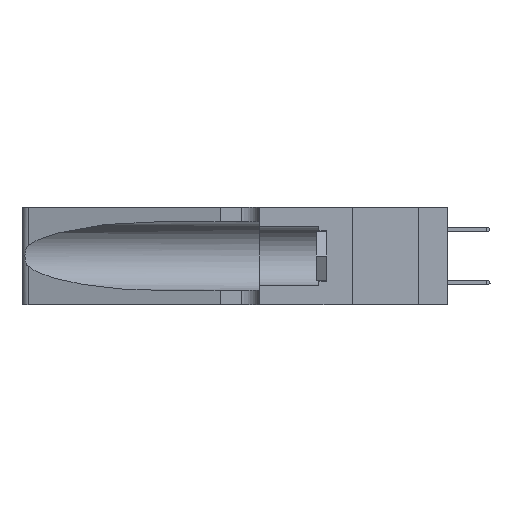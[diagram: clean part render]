
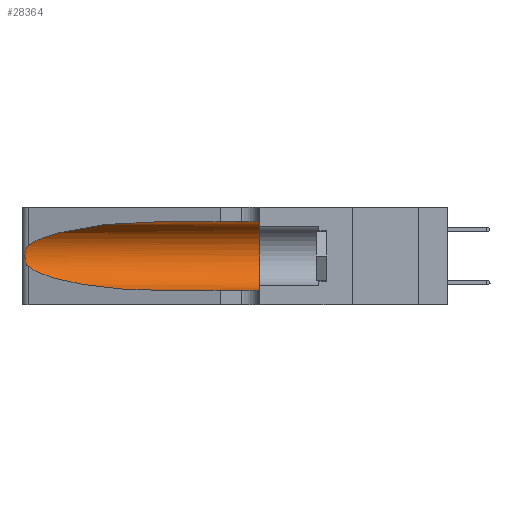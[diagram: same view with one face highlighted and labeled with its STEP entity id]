
A CAD part, left-side view. The second image highlights one B-rep face of the part: STEP entity #28364.
In plain terms, the highlighted cylindrical face has radius 3.308 mm (diameter 6.617 mm), a partial arc.
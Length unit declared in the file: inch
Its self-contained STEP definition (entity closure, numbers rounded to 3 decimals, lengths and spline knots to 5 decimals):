
#409 = CARTESIAN_POINT ( 'NONE',  ( 0.1305, 0.35, 0.31525 ) ) ;
#594 = DIRECTION ( 'NONE',  ( 0., 1., 0. ) ) ;
#695 = ORIENTED_EDGE ( 'NONE', *, *, #9455, .T. ) ;
#910 = AXIS2_PLACEMENT_3D ( 'NONE', #21921, #594, #26947 ) ;
#1210 = CARTESIAN_POINT ( 'NONE',  ( 0.25555, 1.22994, 0.2215 ) ) ;
#2057 = CARTESIAN_POINT ( 'NONE',  ( 0.2373, 1.15595, 0.28018 ) ) ;
#2293 = CARTESIAN_POINT ( 'NONE',  ( 0.1305, 0.72297, 0.31525 ) ) ;
#3059 = VERTEX_POINT ( 'NONE', #32078 ) ;
#3698 = CARTESIAN_POINT ( 'NONE',  ( 0.25487, 1.22718, 0.14631 ) ) ;
#3760 =( BOUNDED_CURVE ( )  B_SPLINE_CURVE ( 3, ( #3698, #6242, #32612, #19324 ),
 .UNSPECIFIED., .F., .F. ) 
 B_SPLINE_CURVE_WITH_KNOTS ( ( 4, 4 ),
 ( 3.44316, 4.71239 ),
 .UNSPECIFIED. ) 
 CURVE ( )  GEOMETRIC_REPRESENTATION_ITEM ( )  RATIONAL_B_SPLINE_CURVE ( ( 1., 0.87, 0.87, 1. ) ) 
 REPRESENTATION_ITEM ( '' )  );
#4035 = CARTESIAN_POINT ( 'NONE',  ( 0.25787, 1.23484, 0.2124 ) ) ;
#4242 = EDGE_CURVE ( 'NONE', #24434, #27949, #31996, .T. ) ;
#4280 = ORIENTED_EDGE ( 'NONE', *, *, #26384, .T. ) ;
#4659 = CARTESIAN_POINT ( 'NONE',  ( 0.25856, 1.23593, 0.16098 ) ) ;
#4873 = CARTESIAN_POINT ( 'NONE',  ( 0.25487, 1.22718, 0.14631 ) ) ;
#4881 = CARTESIAN_POINT ( 'NONE',  ( 0.26075, 1.23896, 0.178 ) ) ;
#5184 = VERTEX_POINT ( 'NONE', #6686 ) ;
#6242 = CARTESIAN_POINT ( 'NONE',  ( 0.2373, 1.15595, 0.08982 ) ) ;
#6261 = EDGE_CURVE ( 'NONE', #5184, #3059, #27499, .T. ) ;
#6686 = CARTESIAN_POINT ( 'NONE',  ( 0.25487, 1.22718, 0.22369 ) ) ;
#7364 = CARTESIAN_POINT ( 'NONE',  ( 0.25789, 1.23486, 0.15765 ) ) ;
#7496 = CARTESIAN_POINT ( 'NONE',  ( 0.1305, 1.61858, 0.05475 ) ) ;
#7864 = DIRECTION ( 'NONE',  ( 0., -1., 0. ) ) ;
#7869 =( BOUNDED_CURVE ( )  B_SPLINE_CURVE ( 3, ( #2293, #9656, #2057, #12314 ),
 .UNSPECIFIED., .F., .T. ) 
 B_SPLINE_CURVE_WITH_KNOTS ( ( 4, 4 ),
 ( 1.5708, 2.84003 ),
 .UNSPECIFIED. ) 
 CURVE ( )  GEOMETRIC_REPRESENTATION_ITEM ( )  RATIONAL_B_SPLINE_CURVE ( ( 1., 0.87, 0.87, 1. ) ) 
 REPRESENTATION_ITEM ( '' )  );
#8290 = LINE ( 'NONE', #7496, #21437 ) ;
#8589 = CARTESIAN_POINT ( 'NONE',  ( 0.1305, 0.72297, 0.31525 ) ) ;
#9378 = CARTESIAN_POINT ( 'NONE',  ( 0.26017, 1.23833, 0.17102 ) ) ;
#9455 = EDGE_CURVE ( 'NONE', #9748, #23220, #8290, .T. ) ;
#9563 = EDGE_CURVE ( 'NONE', #3059, #9748, #3760, .T. ) ;
#9656 = CARTESIAN_POINT ( 'NONE',  ( 0.18966, 0.96281, 0.31525 ) ) ;
#9748 = VERTEX_POINT ( 'NONE', #31173 ) ;
#10279 = DIRECTION ( 'NONE',  ( 0., 0., -1. ) ) ;
#12024 = FACE_OUTER_BOUND ( 'NONE', #28695, .T. ) ;
#12314 = CARTESIAN_POINT ( 'NONE',  ( 0.25487, 1.22718, 0.22369 ) ) ;
#12777 = DIRECTION ( 'NONE',  ( 0., -1., 0. ) ) ;
#13258 = ORIENTED_EDGE ( 'NONE', *, *, #4242, .F. ) ;
#13897 = ORIENTED_EDGE ( 'NONE', *, *, #9563, .T. ) ;
#17250 = CARTESIAN_POINT ( 'NONE',  ( 0.25854, 1.2359, 0.20912 ) ) ;
#17849 = CARTESIAN_POINT ( 'NONE',  ( 0.25555, 1.22993, 0.14849 ) ) ;
#19324 = CARTESIAN_POINT ( 'NONE',  ( 0.1305, 0.72297, 0.05475 ) ) ;
#20195 = CIRCLE ( 'NONE', #910, 0.13025 ) ;
#20371 = CARTESIAN_POINT ( 'NONE',  ( 0.26075, 1.23896, 0.19203 ) ) ;
#20707 = CARTESIAN_POINT ( 'NONE',  ( 0.1305, 1.61858, 0.31525 ) ) ;
#21437 = VECTOR ( 'NONE', #12777, 39.37008 ) ;
#21632 = CARTESIAN_POINT ( 'NONE',  ( 0.1305, 0.35, 0.05475 ) ) ;
#21921 = CARTESIAN_POINT ( 'NONE',  ( 0.1305, 0.35, 0.185 ) ) ;
#23220 = VERTEX_POINT ( 'NONE', #21632 ) ;
#23426 = VECTOR ( 'NONE', #30636, 39.37008 ) ;
#23542 = CARTESIAN_POINT ( 'NONE',  ( 0.1305, 1.61858, 0.185 ) ) ;
#24434 = VERTEX_POINT ( 'NONE', #8589 ) ;
#24454 = ORIENTED_EDGE ( 'NONE', *, *, #6261, .T. ) ;
#24687 = AXIS2_PLACEMENT_3D ( 'NONE', #23542, #7864, #10279 ) ;
#25506 = CARTESIAN_POINT ( 'NONE',  ( 0.25639, 1.23186, 0.15144 ) ) ;
#26384 = EDGE_CURVE ( 'NONE', #24434, #5184, #7869, .T. ) ;
#26394 = CYLINDRICAL_SURFACE ( 'NONE', #24687, 0.13025 ) ;
#26947 = DIRECTION ( 'NONE',  ( 0., 0., 1. ) ) ;
#27499 = B_SPLINE_CURVE_WITH_KNOTS ( 'NONE', 3,
 ( #30056, #1210, #27541, #4035, #17250, #30672, #20371, #4881, #9378, #4659, #7364, #25506, #17849, #4873 ),
 .UNSPECIFIED., .F., .F.,
 ( 4, 2, 2, 2, 2, 2, 4 ),
 ( 0., 0.00027, 0.00053, 0.00107, 0.0016, 0.00187, 0.00214 ),
 .UNSPECIFIED. ) ;
#27541 = CARTESIAN_POINT ( 'NONE',  ( 0.25639, 1.23184, 0.21858 ) ) ;
#27949 = VERTEX_POINT ( 'NONE', #409 ) ;
#28364 = ADVANCED_FACE ( 'NONE', ( #12024 ), #26394, .F. ) ;
#28695 = EDGE_LOOP ( 'NONE', ( #4280, #24454, #13897, #695, #32352, #13258 ) ) ;
#30056 = CARTESIAN_POINT ( 'NONE',  ( 0.25487, 1.22718, 0.22369 ) ) ;
#30636 = DIRECTION ( 'NONE',  ( 0., -1., 0. ) ) ;
#30672 = CARTESIAN_POINT ( 'NONE',  ( 0.26018, 1.23835, 0.19895 ) ) ;
#31173 = CARTESIAN_POINT ( 'NONE',  ( 0.1305, 0.72297, 0.05475 ) ) ;
#31996 = LINE ( 'NONE', #20707, #23426 ) ;
#32078 = CARTESIAN_POINT ( 'NONE',  ( 0.25487, 1.22718, 0.14631 ) ) ;
#32352 = ORIENTED_EDGE ( 'NONE', *, *, #33894, .F. ) ;
#32612 = CARTESIAN_POINT ( 'NONE',  ( 0.18966, 0.96281, 0.05475 ) ) ;
#33894 = EDGE_CURVE ( 'NONE', #27949, #23220, #20195, .T. ) ;
